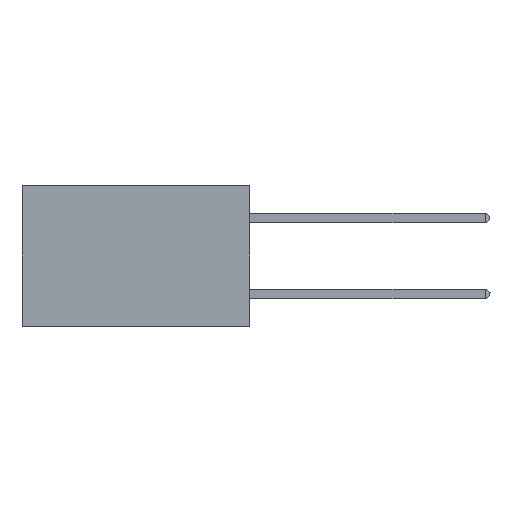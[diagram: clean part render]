
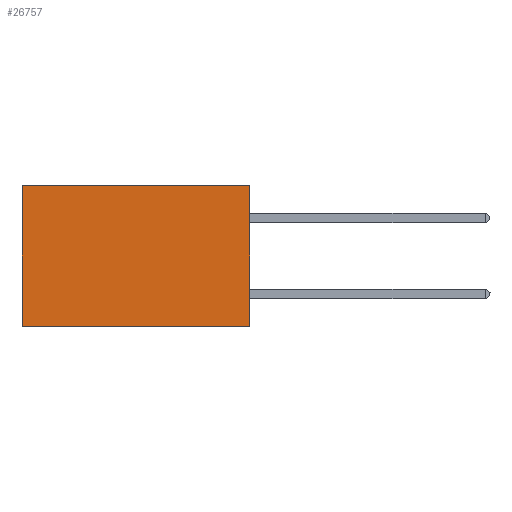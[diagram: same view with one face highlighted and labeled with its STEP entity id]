
A CAD part, left-side view. The second image highlights one B-rep face of the part: STEP entity #26757.
In plain terms, the highlighted planar face has unit normal (-1, 0, 0).
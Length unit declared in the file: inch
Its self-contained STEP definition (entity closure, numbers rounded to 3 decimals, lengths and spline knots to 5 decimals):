
#931 = LINE ( 'NONE', #14718, #27571 ) ;
#3108 = LINE ( 'NONE', #24729, #35399 ) ;
#3840 = EDGE_CURVE ( 'NONE', #10262, #19312, #29038, .T. ) ;
#5985 = VERTEX_POINT ( 'NONE', #40414 ) ;
#6762 = CARTESIAN_POINT ( 'NONE',  ( 0.2875, 0., 0. ) ) ;
#10109 = DIRECTION ( 'NONE',  ( 1., 0., 0. ) ) ;
#10262 = VERTEX_POINT ( 'NONE', #22564 ) ;
#10283 = VECTOR ( 'NONE', #36376, 39.37008 ) ;
#10753 = EDGE_LOOP ( 'NONE', ( #42794, #28983, #33360, #31417 ) ) ;
#12952 = DIRECTION ( 'NONE',  ( 0., 0., -1. ) ) ;
#14307 = VECTOR ( 'NONE', #12952, 39.37008 ) ;
#14718 = CARTESIAN_POINT ( 'NONE',  ( 0.2875, 0.6, 0. ) ) ;
#14793 = FACE_OUTER_BOUND ( 'NONE', #10753, .T. ) ;
#16020 = CARTESIAN_POINT ( 'NONE',  ( 0.2875, 0., -0.37 ) ) ;
#18475 = DIRECTION ( 'NONE',  ( 0., 1., 0. ) ) ;
#19312 = VERTEX_POINT ( 'NONE', #25905 ) ;
#19968 = PLANE ( 'NONE',  #37726 ) ;
#20700 = CARTESIAN_POINT ( 'NONE',  ( 0.2875, 0., 0. ) ) ;
#22564 = CARTESIAN_POINT ( 'NONE',  ( 0.2875, 0., -0.37 ) ) ;
#24729 = CARTESIAN_POINT ( 'NONE',  ( 0.2875, 0., 0. ) ) ;
#25204 = LINE ( 'NONE', #42021, #14307 ) ;
#25905 = CARTESIAN_POINT ( 'NONE',  ( 0.2875, 0.6, -0.37 ) ) ;
#26757 = ADVANCED_FACE ( 'NONE', ( #14793 ), #19968, .F. ) ;
#26976 = DIRECTION ( 'NONE',  ( 0., 0., -1. ) ) ;
#27571 = VECTOR ( 'NONE', #34676, 39.37008 ) ;
#28801 = VERTEX_POINT ( 'NONE', #20700 ) ;
#28858 = EDGE_CURVE ( 'NONE', #28801, #5985, #3108, .T. ) ;
#28983 = ORIENTED_EDGE ( 'NONE', *, *, #3840, .F. ) ;
#29038 = LINE ( 'NONE', #16020, #10283 ) ;
#31417 = ORIENTED_EDGE ( 'NONE', *, *, #28858, .T. ) ;
#32909 = EDGE_CURVE ( 'NONE', #5985, #19312, #931, .T. ) ;
#33360 = ORIENTED_EDGE ( 'NONE', *, *, #40161, .F. ) ;
#34676 = DIRECTION ( 'NONE',  ( 0., 0., -1. ) ) ;
#35399 = VECTOR ( 'NONE', #18475, 39.37008 ) ;
#36376 = DIRECTION ( 'NONE',  ( 0., 1., 0. ) ) ;
#37726 = AXIS2_PLACEMENT_3D ( 'NONE', #6762, #10109, #26976 ) ;
#40161 = EDGE_CURVE ( 'NONE', #28801, #10262, #25204, .T. ) ;
#40414 = CARTESIAN_POINT ( 'NONE',  ( 0.2875, 0.6, 0. ) ) ;
#42021 = CARTESIAN_POINT ( 'NONE',  ( 0.2875, 0., 0. ) ) ;
#42794 = ORIENTED_EDGE ( 'NONE', *, *, #32909, .T. ) ;
